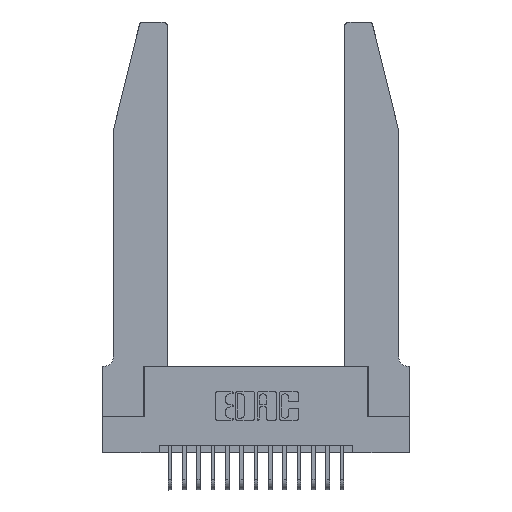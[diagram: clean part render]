
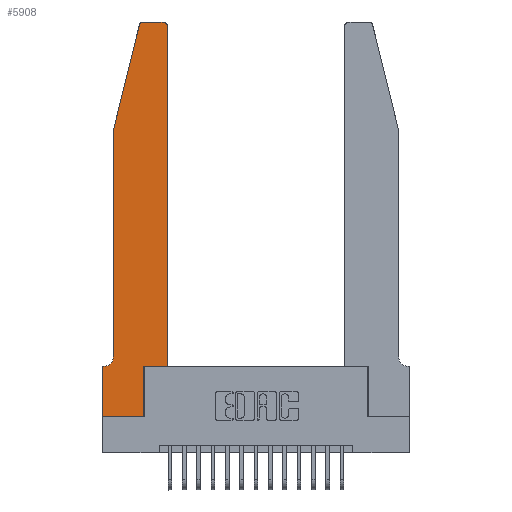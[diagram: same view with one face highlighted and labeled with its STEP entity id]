
A CAD part, top view. The second image highlights one B-rep face of the part: STEP entity #5908.
In plain terms, the highlighted planar face has unit normal (0, 0, 1).
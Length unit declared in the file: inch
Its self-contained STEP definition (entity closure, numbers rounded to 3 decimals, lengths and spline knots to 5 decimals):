
#543 = EDGE_CURVE ( 'NONE', #13712, #12242, #15635, .T. ) ;
#592 = VERTEX_POINT ( 'NONE', #13730 ) ;
#616 = LINE ( 'NONE', #15240, #15903 ) ;
#701 = FACE_OUTER_BOUND ( 'NONE', #13280, .T. ) ;
#846 = CARTESIAN_POINT ( 'NONE',  ( 0., 0.35, 0.37 ) ) ;
#1173 = EDGE_CURVE ( 'NONE', #14221, #10197, #13846, .T. ) ;
#1610 = CARTESIAN_POINT ( 'NONE',  ( 0.4205, 2.72, 0.37 ) ) ;
#1638 = DIRECTION ( 'NONE',  ( 0., 0., 1. ) ) ;
#1714 = ORIENTED_EDGE ( 'NONE', *, *, #4452, .T. ) ;
#2025 = DIRECTION ( 'NONE',  ( 1., 0., 0. ) ) ;
#2897 = CARTESIAN_POINT ( 'NONE',  ( 0., 0.35, 0.37 ) ) ;
#2955 = ORIENTED_EDGE ( 'NONE', *, *, #4020, .T. ) ;
#2984 = CARTESIAN_POINT ( 'NONE',  ( 0.0755, 0.42, 0.37 ) ) ;
#3087 = DIRECTION ( 'NONE',  ( 1., 0., 0. ) ) ;
#3332 = CARTESIAN_POINT ( 'NONE',  ( 0.4205, 2.75, 0.37 ) ) ;
#3403 = ORIENTED_EDGE ( 'NONE', *, *, #18505, .T. ) ;
#3477 = VERTEX_POINT ( 'NONE', #5007 ) ;
#3506 = CARTESIAN_POINT ( 'NONE',  ( 0., 0., 0.37 ) ) ;
#3995 = CIRCLE ( 'NONE', #7548, 0.03 ) ;
#4020 = EDGE_CURVE ( 'NONE', #7526, #6406, #3995, .T. ) ;
#4452 = EDGE_CURVE ( 'NONE', #12242, #14221, #15784, .T. ) ;
#4900 = CARTESIAN_POINT ( 'NONE',  ( 0.0755, 2., 0.37 ) ) ;
#5007 = CARTESIAN_POINT ( 'NONE',  ( 0.4505, 2.72, 0.37 ) ) ;
#5098 = VECTOR ( 'NONE', #6822, 39.37008 ) ;
#5247 = ORIENTED_EDGE ( 'NONE', *, *, #13440, .T. ) ;
#5668 = ORIENTED_EDGE ( 'NONE', *, *, #12301, .T. ) ;
#5908 = ADVANCED_FACE ( 'NONE', ( #701 ), #11118, .T. ) ;
#6406 = VERTEX_POINT ( 'NONE', #17938 ) ;
#6538 = LINE ( 'NONE', #8503, #17374 ) ;
#6822 = DIRECTION ( 'NONE',  ( 0., 1., 0. ) ) ;
#6886 = ORIENTED_EDGE ( 'NONE', *, *, #12164, .T. ) ;
#7465 = VERTEX_POINT ( 'NONE', #3332 ) ;
#7526 = VERTEX_POINT ( 'NONE', #14876 ) ;
#7548 = AXIS2_PLACEMENT_3D ( 'NONE', #10331, #1638, #11753 ) ;
#8285 = VECTOR ( 'NONE', #8638, 39.37008 ) ;
#8302 = LINE ( 'NONE', #12115, #15797 ) ;
#8323 = DIRECTION ( 'NONE',  ( 1., 0., 0. ) ) ;
#8324 = AXIS2_PLACEMENT_3D ( 'NONE', #846, #16750, #8323 ) ;
#8503 = CARTESIAN_POINT ( 'NONE',  ( 0.2605, 2.75, 0.37 ) ) ;
#8638 = DIRECTION ( 'NONE',  ( -1., 0., 0. ) ) ;
#9143 = VERTEX_POINT ( 'NONE', #4900 ) ;
#9382 = VERTEX_POINT ( 'NONE', #16769 ) ;
#9795 = CARTESIAN_POINT ( 'NONE',  ( 0., 0., 0.37 ) ) ;
#9941 = CARTESIAN_POINT ( 'NONE',  ( 0.0755, 2., 0.37 ) ) ;
#10036 = ORIENTED_EDGE ( 'NONE', *, *, #1173, .T. ) ;
#10197 = VERTEX_POINT ( 'NONE', #9795 ) ;
#10306 = EDGE_CURVE ( 'NONE', #10197, #10875, #17388, .T. ) ;
#10331 = CARTESIAN_POINT ( 'NONE',  ( 0.284, 2.72, 0.37 ) ) ;
#10511 = ORIENTED_EDGE ( 'NONE', *, *, #10306, .T. ) ;
#10685 = DIRECTION ( 'NONE',  ( 0., 0., -1. ) ) ;
#10756 = DIRECTION ( 'NONE',  ( -1., 0., 0. ) ) ;
#10875 = VERTEX_POINT ( 'NONE', #11334 ) ;
#11118 = PLANE ( 'NONE',  #8324 ) ;
#11133 = CARTESIAN_POINT ( 'NONE',  ( 0.2865, 0.35, 0.37 ) ) ;
#11304 = DIRECTION ( 'NONE',  ( -0.239, -0.971, 0. ) ) ;
#11334 = CARTESIAN_POINT ( 'NONE',  ( 0.2865, 0., 0.37 ) ) ;
#11463 = CARTESIAN_POINT ( 'NONE',  ( 0., 0., 0.37 ) ) ;
#11464 = CIRCLE ( 'NONE', #16840, 0.03 ) ;
#11550 = CARTESIAN_POINT ( 'NONE',  ( 0.0055, 0.42, 0.37 ) ) ;
#11725 = DIRECTION ( 'NONE',  ( 0., 0., 1. ) ) ;
#11753 = DIRECTION ( 'NONE',  ( 1., 0., 0. ) ) ;
#12111 = EDGE_CURVE ( 'NONE', #9382, #592, #8302, .T. ) ;
#12115 = CARTESIAN_POINT ( 'NONE',  ( 0.4505, 0.35, 0.37 ) ) ;
#12164 = EDGE_CURVE ( 'NONE', #592, #3477, #18176, .T. ) ;
#12242 = VERTEX_POINT ( 'NONE', #13761 ) ;
#12301 = EDGE_CURVE ( 'NONE', #10875, #9382, #16443, .T. ) ;
#12863 = DIRECTION ( 'NONE',  ( 1., 0., 0. ) ) ;
#13114 = ORIENTED_EDGE ( 'NONE', *, *, #15849, .T. ) ;
#13280 = EDGE_LOOP ( 'NONE', ( #14573, #2955, #3403, #5247, #17705, #1714, #10036, #10511, #5668, #16235, #6886, #13114 ) ) ;
#13440 = EDGE_CURVE ( 'NONE', #9143, #13712, #616, .T. ) ;
#13661 = VECTOR ( 'NONE', #12863, 39.37008 ) ;
#13712 = VERTEX_POINT ( 'NONE', #2984 ) ;
#13730 = CARTESIAN_POINT ( 'NONE',  ( 0.4505, 0.35, 0.37 ) ) ;
#13761 = CARTESIAN_POINT ( 'NONE',  ( 0.0055, 0.35, 0.37 ) ) ;
#13846 = LINE ( 'NONE', #3506, #14282 ) ;
#14165 = VECTOR ( 'NONE', #11304, 39.37008 ) ;
#14221 = VERTEX_POINT ( 'NONE', #2897 ) ;
#14282 = VECTOR ( 'NONE', #14937, 39.37008 ) ;
#14294 = AXIS2_PLACEMENT_3D ( 'NONE', #11550, #10685, #10756 ) ;
#14464 = VECTOR ( 'NONE', #17860, 39.37008 ) ;
#14573 = ORIENTED_EDGE ( 'NONE', *, *, #15697, .T. ) ;
#14876 = CARTESIAN_POINT ( 'NONE',  ( 0.284, 2.75, 0.37 ) ) ;
#14937 = DIRECTION ( 'NONE',  ( 0., -1., 0. ) ) ;
#15240 = CARTESIAN_POINT ( 'NONE',  ( 0.0755, 2., 0.37 ) ) ;
#15635 = CIRCLE ( 'NONE', #14294, 0.07 ) ;
#15697 = EDGE_CURVE ( 'NONE', #7465, #7526, #6538, .T. ) ;
#15784 = LINE ( 'NONE', #17054, #8285 ) ;
#15797 = VECTOR ( 'NONE', #2025, 39.37008 ) ;
#15849 = EDGE_CURVE ( 'NONE', #3477, #7465, #11464, .T. ) ;
#15903 = VECTOR ( 'NONE', #16626, 39.37008 ) ;
#16235 = ORIENTED_EDGE ( 'NONE', *, *, #12111, .T. ) ;
#16398 = CARTESIAN_POINT ( 'NONE',  ( 0.4505, 0.35, 0.37 ) ) ;
#16443 = LINE ( 'NONE', #11133, #5098 ) ;
#16626 = DIRECTION ( 'NONE',  ( 0., -1., 0. ) ) ;
#16750 = DIRECTION ( 'NONE',  ( 0., 0., 1. ) ) ;
#16769 = CARTESIAN_POINT ( 'NONE',  ( 0.2865, 0.35, 0.37 ) ) ;
#16840 = AXIS2_PLACEMENT_3D ( 'NONE', #1610, #11725, #3087 ) ;
#17054 = CARTESIAN_POINT ( 'NONE',  ( 0.0755, 0.35, 0.37 ) ) ;
#17374 = VECTOR ( 'NONE', #18317, 39.37008 ) ;
#17388 = LINE ( 'NONE', #11463, #13661 ) ;
#17705 = ORIENTED_EDGE ( 'NONE', *, *, #543, .T. ) ;
#17860 = DIRECTION ( 'NONE',  ( 0., 1., 0. ) ) ;
#17938 = CARTESIAN_POINT ( 'NONE',  ( 0.25487, 2.72718, 0.37 ) ) ;
#18176 = LINE ( 'NONE', #16398, #14464 ) ;
#18308 = LINE ( 'NONE', #9941, #14165 ) ;
#18317 = DIRECTION ( 'NONE',  ( -1., 0., 0. ) ) ;
#18505 = EDGE_CURVE ( 'NONE', #6406, #9143, #18308, .T. ) ;
